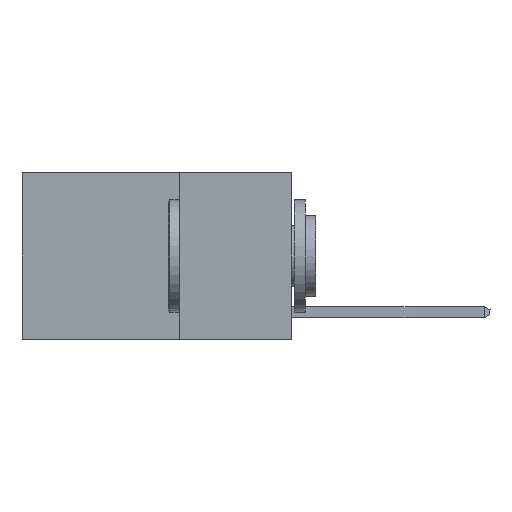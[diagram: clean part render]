
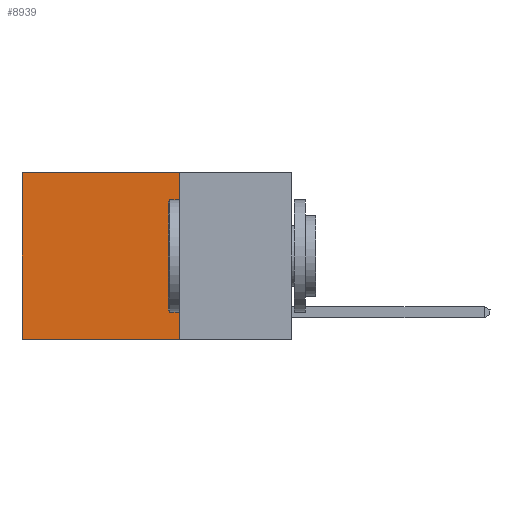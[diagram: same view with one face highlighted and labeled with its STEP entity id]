
A CAD part, left-side view. The second image highlights one B-rep face of the part: STEP entity #8939.
In plain terms, the highlighted planar face has unit normal (-1, 0, 0).
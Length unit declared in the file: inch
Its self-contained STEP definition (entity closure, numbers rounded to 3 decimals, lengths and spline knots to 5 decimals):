
#1049 = CARTESIAN_POINT ( 'NONE',  ( 0.2625, 0.25, 0. ) ) ;
#1075 = CARTESIAN_POINT ( 'NONE',  ( 0.2625, 0.6, -0.37 ) ) ;
#1602 = LINE ( 'NONE', #9855, #12702 ) ;
#2570 = VECTOR ( 'NONE', #3417, 39.37008 ) ;
#3417 = DIRECTION ( 'NONE',  ( 0., 0., -1. ) ) ;
#4385 = VECTOR ( 'NONE', #26025, 39.37008 ) ;
#4752 = LINE ( 'NONE', #27238, #22118 ) ;
#5145 = DIRECTION ( 'NONE',  ( 0., 0., -1. ) ) ;
#8939 = ADVANCED_FACE ( 'NONE', ( #13028 ), #16939, .F. ) ;
#9855 = CARTESIAN_POINT ( 'NONE',  ( 0.2625, 0.6, 0. ) ) ;
#10679 = LINE ( 'NONE', #11907, #4385 ) ;
#10695 = VERTEX_POINT ( 'NONE', #16239 ) ;
#10715 = DIRECTION ( 'NONE',  ( 0., 1., 0. ) ) ;
#10723 = VERTEX_POINT ( 'NONE', #18687 ) ;
#10805 = EDGE_CURVE ( 'NONE', #10723, #20453, #10679, .T. ) ;
#11907 = CARTESIAN_POINT ( 'NONE',  ( 0.2625, 0.25, 0. ) ) ;
#12194 = CARTESIAN_POINT ( 'NONE',  ( 0.2625, 0.25, 0. ) ) ;
#12328 = ORIENTED_EDGE ( 'NONE', *, *, #25912, .F. ) ;
#12702 = VECTOR ( 'NONE', #16877, 39.37008 ) ;
#13028 = FACE_OUTER_BOUND ( 'NONE', #14681, .T. ) ;
#13536 = EDGE_CURVE ( 'NONE', #20453, #18971, #1602, .T. ) ;
#14681 = EDGE_LOOP ( 'NONE', ( #25971, #17120, #12328, #18594 ) ) ;
#16239 = CARTESIAN_POINT ( 'NONE',  ( 0.2625, 0.25, -0.37 ) ) ;
#16281 = CARTESIAN_POINT ( 'NONE',  ( 0.2625, 0.6, 0. ) ) ;
#16877 = DIRECTION ( 'NONE',  ( 0., 0., -1. ) ) ;
#16939 = PLANE ( 'NONE',  #24127 ) ;
#17120 = ORIENTED_EDGE ( 'NONE', *, *, #26305, .F. ) ;
#18594 = ORIENTED_EDGE ( 'NONE', *, *, #10805, .T. ) ;
#18687 = CARTESIAN_POINT ( 'NONE',  ( 0.2625, 0.25, 0. ) ) ;
#18971 = VERTEX_POINT ( 'NONE', #1075 ) ;
#19294 = DIRECTION ( 'NONE',  ( 1., 0., 0. ) ) ;
#20453 = VERTEX_POINT ( 'NONE', #16281 ) ;
#21398 = LINE ( 'NONE', #1049, #2570 ) ;
#22118 = VECTOR ( 'NONE', #10715, 39.37008 ) ;
#24127 = AXIS2_PLACEMENT_3D ( 'NONE', #12194, #19294, #5145 ) ;
#25912 = EDGE_CURVE ( 'NONE', #10723, #10695, #21398, .T. ) ;
#25971 = ORIENTED_EDGE ( 'NONE', *, *, #13536, .T. ) ;
#26025 = DIRECTION ( 'NONE',  ( 0., 1., 0. ) ) ;
#26305 = EDGE_CURVE ( 'NONE', #10695, #18971, #4752, .T. ) ;
#27238 = CARTESIAN_POINT ( 'NONE',  ( 0.2625, 0.25, -0.37 ) ) ;
